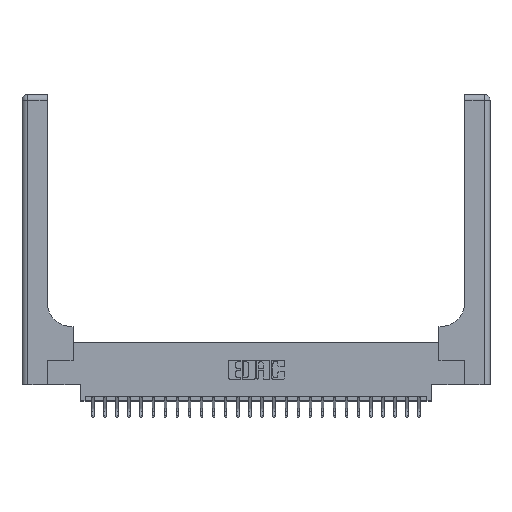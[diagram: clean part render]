
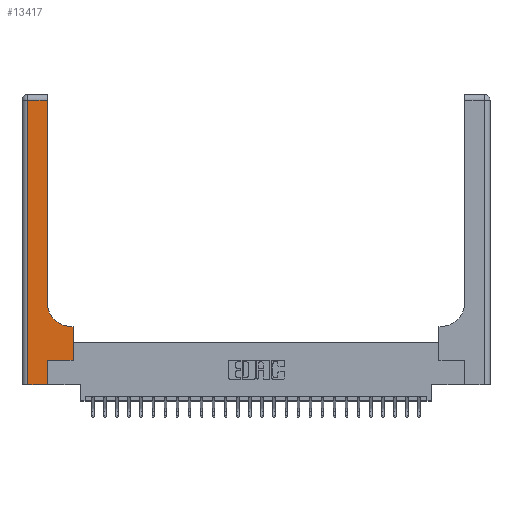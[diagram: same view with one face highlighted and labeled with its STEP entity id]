
A CAD part, top view. The second image highlights one B-rep face of the part: STEP entity #13417.
In plain terms, the highlighted planar face has unit normal (0, 0, 1).
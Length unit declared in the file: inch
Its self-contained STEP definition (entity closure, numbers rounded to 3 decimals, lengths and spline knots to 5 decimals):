
#86 = CARTESIAN_POINT ( 'NONE',  ( 0.06, 0., 0.37 ) ) ;
#175 = ORIENTED_EDGE ( 'NONE', *, *, #3850, .T. ) ;
#716 = EDGE_CURVE ( 'NONE', #8483, #12366, #24550, .T. ) ;
#980 = ORIENTED_EDGE ( 'NONE', *, *, #18333, .T. ) ;
#1129 = CARTESIAN_POINT ( 'NONE',  ( 0.26, 0.85, 0.37 ) ) ;
#1141 = ORIENTED_EDGE ( 'NONE', *, *, #8594, .T. ) ;
#1338 = CARTESIAN_POINT ( 'NONE',  ( 0.265, 0.25, 0.37 ) ) ;
#1422 = CARTESIAN_POINT ( 'NONE',  ( 0.528, 0.25, 0.37 ) ) ;
#1469 = EDGE_CURVE ( 'NONE', #24650, #22559, #8457, .T. ) ;
#1474 = CARTESIAN_POINT ( 'NONE',  ( 0.26, 2.94, 0.37 ) ) ;
#1486 = DIRECTION ( 'NONE',  ( 0., 1., 0. ) ) ;
#1749 = EDGE_CURVE ( 'NONE', #22559, #19835, #23300, .T. ) ;
#1916 = LINE ( 'NONE', #5445, #11931 ) ;
#2066 = VECTOR ( 'NONE', #23427, 39.37008 ) ;
#2085 = EDGE_LOOP ( 'NONE', ( #16563, #5193, #11704, #16696, #16714, #1141, #980, #10258, #175 ) ) ;
#2281 = FACE_OUTER_BOUND ( 'NONE', #2085, .T. ) ;
#2345 = EDGE_CURVE ( 'NONE', #10142, #5930, #7388, .T. ) ;
#2553 = CARTESIAN_POINT ( 'NONE',  ( 0.06, 2.94, 0.37 ) ) ;
#2693 = VERTEX_POINT ( 'NONE', #6936 ) ;
#2713 = DIRECTION ( 'NONE',  ( -1., 0., 0. ) ) ;
#2931 = LINE ( 'NONE', #1422, #12957 ) ;
#3850 = EDGE_CURVE ( 'NONE', #5930, #8483, #17308, .T. ) ;
#5193 = ORIENTED_EDGE ( 'NONE', *, *, #7010, .T. ) ;
#5429 = DIRECTION ( 'NONE',  ( 1., 0., 0. ) ) ;
#5445 = CARTESIAN_POINT ( 'NONE',  ( 0.265, 0., 0.37 ) ) ;
#5930 = VERTEX_POINT ( 'NONE', #9308 ) ;
#6004 = EDGE_CURVE ( 'NONE', #19835, #7814, #1916, .T. ) ;
#6936 = CARTESIAN_POINT ( 'NONE',  ( 0.528, 0.25, 0.37 ) ) ;
#7010 = EDGE_CURVE ( 'NONE', #12366, #24650, #18726, .T. ) ;
#7221 = VECTOR ( 'NONE', #5429, 39.37008 ) ;
#7388 = LINE ( 'NONE', #9579, #2066 ) ;
#7814 = VERTEX_POINT ( 'NONE', #1338 ) ;
#8128 = VECTOR ( 'NONE', #2713, 39.37008 ) ;
#8362 = DIRECTION ( 'NONE',  ( 0., 1., 0. ) ) ;
#8457 = LINE ( 'NONE', #17046, #13139 ) ;
#8483 = VERTEX_POINT ( 'NONE', #1129 ) ;
#8594 = EDGE_CURVE ( 'NONE', #7814, #2693, #12555, .T. ) ;
#8629 = CARTESIAN_POINT ( 'NONE',  ( 0.26, 3., 0.37 ) ) ;
#8808 = VECTOR ( 'NONE', #8362, 39.37008 ) ;
#9072 = CARTESIAN_POINT ( 'NONE',  ( 0., 3., 0.37 ) ) ;
#9308 = CARTESIAN_POINT ( 'NONE',  ( 0.51, 0.6, 0.37 ) ) ;
#9579 = CARTESIAN_POINT ( 'NONE',  ( 0.26, 0.6, 0.37 ) ) ;
#9946 = CARTESIAN_POINT ( 'NONE',  ( 0., 0., 0.37 ) ) ;
#10142 = VERTEX_POINT ( 'NONE', #24093 ) ;
#10183 = CARTESIAN_POINT ( 'NONE',  ( 0.51, 0.85, 0.37 ) ) ;
#10258 = ORIENTED_EDGE ( 'NONE', *, *, #2345, .T. ) ;
#11068 = DIRECTION ( 'NONE',  ( -1., 0., 0. ) ) ;
#11704 = ORIENTED_EDGE ( 'NONE', *, *, #1469, .T. ) ;
#11931 = VECTOR ( 'NONE', #1486, 39.37008 ) ;
#12122 = CARTESIAN_POINT ( 'NONE',  ( 0.265, 0., 0.37 ) ) ;
#12199 = DIRECTION ( 'NONE',  ( 1., 0., 0. ) ) ;
#12366 = VERTEX_POINT ( 'NONE', #1474 ) ;
#12555 = LINE ( 'NONE', #23217, #7221 ) ;
#12957 = VECTOR ( 'NONE', #23242, 39.37008 ) ;
#13139 = VECTOR ( 'NONE', #23037, 39.37008 ) ;
#13417 = ADVANCED_FACE ( 'NONE', ( #2281 ), #20955, .F. ) ;
#14187 = AXIS2_PLACEMENT_3D ( 'NONE', #9072, #22913, #11068 ) ;
#14763 = CARTESIAN_POINT ( 'NONE',  ( 0., 2.94, 0.37 ) ) ;
#16563 = ORIENTED_EDGE ( 'NONE', *, *, #716, .T. ) ;
#16696 = ORIENTED_EDGE ( 'NONE', *, *, #1749, .T. ) ;
#16714 = ORIENTED_EDGE ( 'NONE', *, *, #6004, .T. ) ;
#17046 = CARTESIAN_POINT ( 'NONE',  ( 0.06, 3., 0.37 ) ) ;
#17308 = CIRCLE ( 'NONE', #17590, 0.25 ) ;
#17590 = AXIS2_PLACEMENT_3D ( 'NONE', #10183, #24005, #12199 ) ;
#18333 = EDGE_CURVE ( 'NONE', #2693, #10142, #2931, .T. ) ;
#18726 = LINE ( 'NONE', #14763, #8128 ) ;
#19835 = VERTEX_POINT ( 'NONE', #12122 ) ;
#20955 = PLANE ( 'NONE',  #14187 ) ;
#22559 = VERTEX_POINT ( 'NONE', #86 ) ;
#22688 = VECTOR ( 'NONE', #23800, 39.37008 ) ;
#22913 = DIRECTION ( 'NONE',  ( 0., 0., -1. ) ) ;
#23037 = DIRECTION ( 'NONE',  ( 0., -1., 0. ) ) ;
#23217 = CARTESIAN_POINT ( 'NONE',  ( 0.265, 0.25, 0.37 ) ) ;
#23242 = DIRECTION ( 'NONE',  ( 0., 1., 0. ) ) ;
#23300 = LINE ( 'NONE', #9946, #22688 ) ;
#23427 = DIRECTION ( 'NONE',  ( -1., 0., 0. ) ) ;
#23800 = DIRECTION ( 'NONE',  ( 1., 0., 0. ) ) ;
#24005 = DIRECTION ( 'NONE',  ( 0., 0., -1. ) ) ;
#24093 = CARTESIAN_POINT ( 'NONE',  ( 0.528, 0.6, 0.37 ) ) ;
#24550 = LINE ( 'NONE', #8629, #8808 ) ;
#24650 = VERTEX_POINT ( 'NONE', #2553 ) ;
